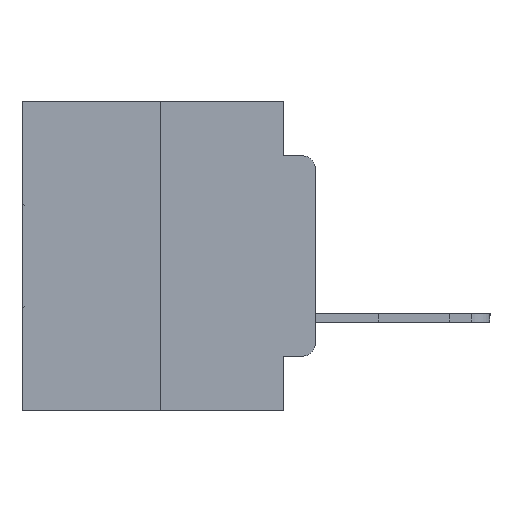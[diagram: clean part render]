
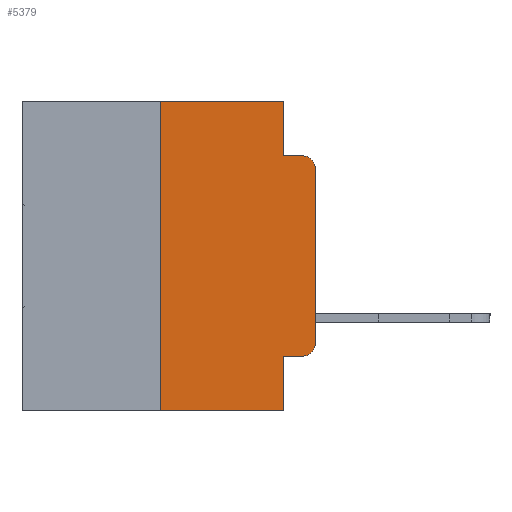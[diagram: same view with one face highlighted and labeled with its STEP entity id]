
A CAD part, left-side view. The second image highlights one B-rep face of the part: STEP entity #5379.
In plain terms, the highlighted planar face has unit normal (-1, 0, 0).
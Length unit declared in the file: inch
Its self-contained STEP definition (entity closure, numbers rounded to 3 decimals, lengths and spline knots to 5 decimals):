
#226 = CARTESIAN_POINT ( 'NONE',  ( 0., 0.051, 0. ) ) ;
#1221 = CARTESIAN_POINT ( 'NONE',  ( 0., 0.051, 0. ) ) ;
#1311 = ORIENTED_EDGE ( 'NONE', *, *, #18827, .T. ) ;
#1453 = VERTEX_POINT ( 'NONE', #16834 ) ;
#1925 = VERTEX_POINT ( 'NONE', #12832 ) ;
#2329 = VECTOR ( 'NONE', #28759, 39.37008 ) ;
#2933 = VERTEX_POINT ( 'NONE', #27605 ) ;
#3084 = VECTOR ( 'NONE', #4556, 39.37008 ) ;
#3508 = EDGE_LOOP ( 'NONE', ( #15229, #22371, #17294, #29388, #6460, #19362, #1311, #20033, #26421, #4565 ) ) ;
#3820 = DIRECTION ( 'NONE',  ( 0., 0., -1. ) ) ;
#3831 = FACE_OUTER_BOUND ( 'NONE', #3508, .T. ) ;
#3970 = DIRECTION ( 'NONE',  ( 0., -1., 0. ) ) ;
#4089 = EDGE_CURVE ( 'NONE', #14744, #24500, #9578, .T. ) ;
#4462 = VERTEX_POINT ( 'NONE', #26404 ) ;
#4473 = EDGE_CURVE ( 'NONE', #28666, #4462, #9233, .T. ) ;
#4556 = DIRECTION ( 'NONE',  ( 0., -1., 0. ) ) ;
#4565 = ORIENTED_EDGE ( 'NONE', *, *, #4473, .T. ) ;
#5229 = CARTESIAN_POINT ( 'NONE',  ( 0., 0.02, -0.4115 ) ) ;
#5276 = DIRECTION ( 'NONE',  ( 0., 0., 1. ) ) ;
#5379 = ADVANCED_FACE ( 'NONE', ( #3831 ), #24138, .F. ) ;
#6460 = ORIENTED_EDGE ( 'NONE', *, *, #4089, .F. ) ;
#7715 = CARTESIAN_POINT ( 'NONE',  ( 0., 0.051, -0.5 ) ) ;
#7877 = VECTOR ( 'NONE', #5276, 39.37008 ) ;
#8631 = VERTEX_POINT ( 'NONE', #7715 ) ;
#8737 = CARTESIAN_POINT ( 'NONE',  ( 0., 0.02, -0.3915 ) ) ;
#9106 = CARTESIAN_POINT ( 'NONE',  ( 0., 0.02, -0.1085 ) ) ;
#9233 = CIRCLE ( 'NONE', #12127, 0.02 ) ;
#9578 = LINE ( 'NONE', #22667, #3084 ) ;
#9631 = LINE ( 'NONE', #11283, #2329 ) ;
#10105 = CARTESIAN_POINT ( 'NONE',  ( 0., 0.25, -0.5 ) ) ;
#10902 = EDGE_CURVE ( 'NONE', #1925, #28666, #15023, .T. ) ;
#11109 = DIRECTION ( 'NONE',  ( 0., 0., -1. ) ) ;
#11176 = LINE ( 'NONE', #14200, #16514 ) ;
#11283 = CARTESIAN_POINT ( 'NONE',  ( 0., 0., 0. ) ) ;
#11474 = DIRECTION ( 'NONE',  ( 0., 0., -1. ) ) ;
#11499 = VECTOR ( 'NONE', #3820, 39.37008 ) ;
#11609 = VERTEX_POINT ( 'NONE', #24997 ) ;
#12127 = AXIS2_PLACEMENT_3D ( 'NONE', #8737, #24351, #11109 ) ;
#12463 = EDGE_CURVE ( 'NONE', #1925, #8631, #22127, .T. ) ;
#12832 = CARTESIAN_POINT ( 'NONE',  ( 0., 0.051, -0.4115 ) ) ;
#13226 = DIRECTION ( 'NONE',  ( 1., 0., 0. ) ) ;
#13971 = EDGE_CURVE ( 'NONE', #27440, #14744, #21304, .T. ) ;
#14200 = CARTESIAN_POINT ( 'NONE',  ( 0., 0.473, -0.5 ) ) ;
#14744 = VERTEX_POINT ( 'NONE', #17459 ) ;
#14966 = VECTOR ( 'NONE', #23495, 39.37008 ) ;
#15023 = LINE ( 'NONE', #27413, #25902 ) ;
#15229 = ORIENTED_EDGE ( 'NONE', *, *, #22767, .T. ) ;
#15501 = EDGE_CURVE ( 'NONE', #24500, #2933, #23227, .T. ) ;
#16282 = CARTESIAN_POINT ( 'NONE',  ( 0., 0.051, 0. ) ) ;
#16514 = VECTOR ( 'NONE', #25292, 39.37008 ) ;
#16834 = CARTESIAN_POINT ( 'NONE',  ( 0., 0.02, -0.0885 ) ) ;
#17294 = ORIENTED_EDGE ( 'NONE', *, *, #18451, .F. ) ;
#17459 = CARTESIAN_POINT ( 'NONE',  ( 0., 0.25, 0. ) ) ;
#17553 = LINE ( 'NONE', #20110, #28307 ) ;
#18451 = EDGE_CURVE ( 'NONE', #2933, #1453, #17553, .T. ) ;
#18827 = EDGE_CURVE ( 'NONE', #27440, #8631, #11176, .T. ) ;
#19064 = CARTESIAN_POINT ( 'NONE',  ( 0., 0.25, 0. ) ) ;
#19362 = ORIENTED_EDGE ( 'NONE', *, *, #13971, .F. ) ;
#19918 = EDGE_CURVE ( 'NONE', #11609, #1453, #26939, .T. ) ;
#20033 = ORIENTED_EDGE ( 'NONE', *, *, #12463, .F. ) ;
#20110 = CARTESIAN_POINT ( 'NONE',  ( 0., 0.051, -0.0885 ) ) ;
#21304 = LINE ( 'NONE', #19064, #7877 ) ;
#22127 = LINE ( 'NONE', #226, #14966 ) ;
#22371 = ORIENTED_EDGE ( 'NONE', *, *, #19918, .T. ) ;
#22667 = CARTESIAN_POINT ( 'NONE',  ( 0., 0.473, 0. ) ) ;
#22767 = EDGE_CURVE ( 'NONE', #4462, #11609, #9631, .T. ) ;
#23094 = DIRECTION ( 'NONE',  ( 0., -1., 0. ) ) ;
#23227 = LINE ( 'NONE', #1221, #11499 ) ;
#23495 = DIRECTION ( 'NONE',  ( 0., 0., -1. ) ) ;
#24138 = PLANE ( 'NONE',  #27503 ) ;
#24249 = AXIS2_PLACEMENT_3D ( 'NONE', #9106, #24694, #11474 ) ;
#24351 = DIRECTION ( 'NONE',  ( -1., 0., 0. ) ) ;
#24500 = VERTEX_POINT ( 'NONE', #16282 ) ;
#24694 = DIRECTION ( 'NONE',  ( -1., 0., 0. ) ) ;
#24997 = CARTESIAN_POINT ( 'NONE',  ( 0., 0., -0.1085 ) ) ;
#25292 = DIRECTION ( 'NONE',  ( 0., -1., 0. ) ) ;
#25902 = VECTOR ( 'NONE', #23094, 39.37008 ) ;
#26298 = CARTESIAN_POINT ( 'NONE',  ( 0., 0.473, 0. ) ) ;
#26404 = CARTESIAN_POINT ( 'NONE',  ( 0., 0., -0.3915 ) ) ;
#26421 = ORIENTED_EDGE ( 'NONE', *, *, #10902, .T. ) ;
#26939 = CIRCLE ( 'NONE', #24249, 0.02 ) ;
#27413 = CARTESIAN_POINT ( 'NONE',  ( 0., 0.051, -0.4115 ) ) ;
#27440 = VERTEX_POINT ( 'NONE', #10105 ) ;
#27503 = AXIS2_PLACEMENT_3D ( 'NONE', #26298, #13226, #28414 ) ;
#27605 = CARTESIAN_POINT ( 'NONE',  ( 0., 0.051, -0.0885 ) ) ;
#28307 = VECTOR ( 'NONE', #3970, 39.37008 ) ;
#28414 = DIRECTION ( 'NONE',  ( 0., 0., -1. ) ) ;
#28666 = VERTEX_POINT ( 'NONE', #5229 ) ;
#28759 = DIRECTION ( 'NONE',  ( 0., 0., 1. ) ) ;
#29388 = ORIENTED_EDGE ( 'NONE', *, *, #15501, .F. ) ;
